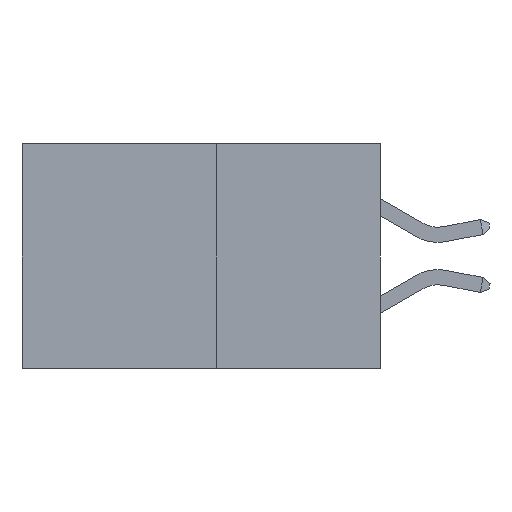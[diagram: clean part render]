
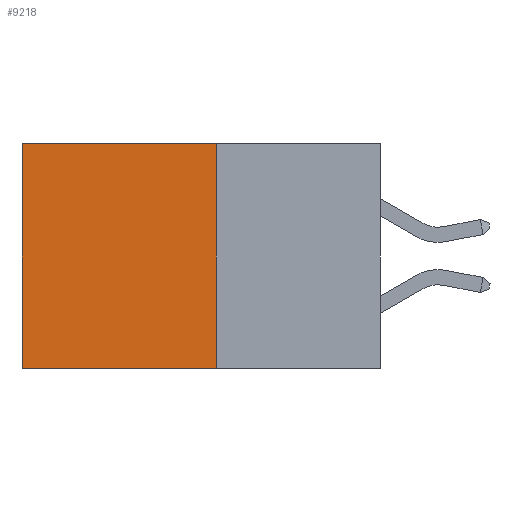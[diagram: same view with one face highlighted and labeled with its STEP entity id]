
A CAD part, left-side view. The second image highlights one B-rep face of the part: STEP entity #9218.
In plain terms, the highlighted planar face has unit normal (-1, 0, 0).
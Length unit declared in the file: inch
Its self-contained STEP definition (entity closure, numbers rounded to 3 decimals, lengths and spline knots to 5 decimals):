
#639 = VERTEX_POINT ( 'NONE', #5773 ) ;
#946 = VECTOR ( 'NONE', #5701, 39.37008 ) ;
#1493 = LINE ( 'NONE', #3991, #5931 ) ;
#1658 = VERTEX_POINT ( 'NONE', #14759 ) ;
#1671 = EDGE_CURVE ( 'NONE', #23296, #639, #1493, .T. ) ;
#2548 = ORIENTED_EDGE ( 'NONE', *, *, #22299, .F. ) ;
#2596 = LINE ( 'NONE', #14930, #16369 ) ;
#3545 = CARTESIAN_POINT ( 'NONE',  ( 0.277, 0.27, 0. ) ) ;
#3968 = LINE ( 'NONE', #18986, #23116 ) ;
#3991 = CARTESIAN_POINT ( 'NONE',  ( 0.277, 0.27, 0. ) ) ;
#4206 = VERTEX_POINT ( 'NONE', #16809 ) ;
#4775 = AXIS2_PLACEMENT_3D ( 'NONE', #12695, #12255, #12202 ) ;
#5701 = DIRECTION ( 'NONE',  ( 0., 0., -1. ) ) ;
#5773 = CARTESIAN_POINT ( 'NONE',  ( 0.277, 0.59, 0. ) ) ;
#5931 = VECTOR ( 'NONE', #20602, 39.37008 ) ;
#6796 = ORIENTED_EDGE ( 'NONE', *, *, #9021, .F. ) ;
#9021 = EDGE_CURVE ( 'NONE', #23296, #1658, #2596, .T. ) ;
#9218 = ADVANCED_FACE ( 'NONE', ( #17225 ), #12312, .F. ) ;
#12202 = DIRECTION ( 'NONE',  ( 0., 0., -1. ) ) ;
#12255 = DIRECTION ( 'NONE',  ( 1., 0., 0. ) ) ;
#12312 = PLANE ( 'NONE',  #4775 ) ;
#12695 = CARTESIAN_POINT ( 'NONE',  ( 0.277, 0.27, -0.37 ) ) ;
#14759 = CARTESIAN_POINT ( 'NONE',  ( 0.277, 0.27, -0.37 ) ) ;
#14818 = DIRECTION ( 'NONE',  ( 0., 0., -1. ) ) ;
#14930 = CARTESIAN_POINT ( 'NONE',  ( 0.277, 0.27, -0.37 ) ) ;
#14998 = CARTESIAN_POINT ( 'NONE',  ( 0.277, 0.59, -0.37 ) ) ;
#15903 = LINE ( 'NONE', #14998, #946 ) ;
#16067 = ORIENTED_EDGE ( 'NONE', *, *, #1671, .T. ) ;
#16369 = VECTOR ( 'NONE', #14818, 39.37008 ) ;
#16718 = EDGE_LOOP ( 'NONE', ( #22284, #2548, #6796, #16067 ) ) ;
#16809 = CARTESIAN_POINT ( 'NONE',  ( 0.277, 0.59, -0.37 ) ) ;
#17225 = FACE_OUTER_BOUND ( 'NONE', #16718, .T. ) ;
#17936 = EDGE_CURVE ( 'NONE', #639, #4206, #15903, .T. ) ;
#18986 = CARTESIAN_POINT ( 'NONE',  ( 0.277, 0.27, -0.37 ) ) ;
#20602 = DIRECTION ( 'NONE',  ( 0., 1., 0. ) ) ;
#22284 = ORIENTED_EDGE ( 'NONE', *, *, #17936, .T. ) ;
#22299 = EDGE_CURVE ( 'NONE', #1658, #4206, #3968, .T. ) ;
#22680 = DIRECTION ( 'NONE',  ( 0., 1., 0. ) ) ;
#23116 = VECTOR ( 'NONE', #22680, 39.37008 ) ;
#23296 = VERTEX_POINT ( 'NONE', #3545 ) ;
